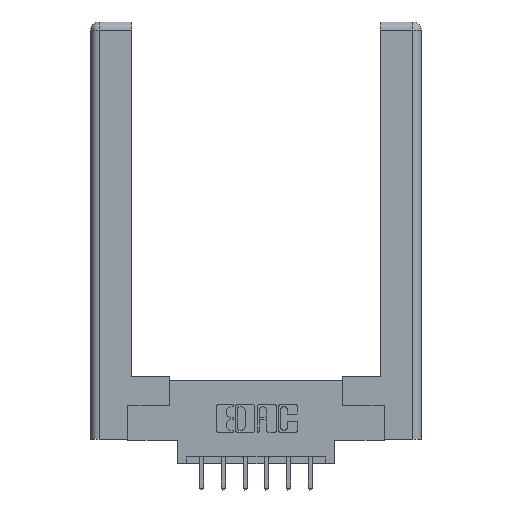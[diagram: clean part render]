
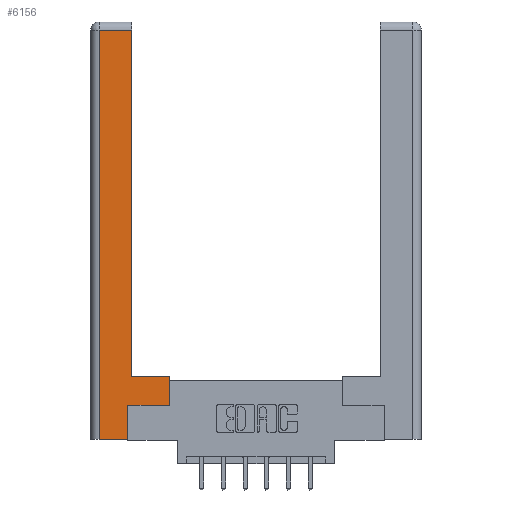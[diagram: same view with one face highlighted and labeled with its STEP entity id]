
A CAD part, top view. The second image highlights one B-rep face of the part: STEP entity #6156.
In plain terms, the highlighted planar face has unit normal (0, 0, 1).
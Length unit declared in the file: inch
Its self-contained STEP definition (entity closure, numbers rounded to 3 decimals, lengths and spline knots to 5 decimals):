
#285 = CARTESIAN_POINT ( 'NONE',  ( 0.565, 0.45, 0. ) ) ;
#335 = VERTEX_POINT ( 'NONE', #6458 ) ;
#541 = EDGE_LOOP ( 'NONE', ( #3999, #8343, #9172, #4169, #6907, #8068, #10866, #2888 ) ) ;
#599 = PLANE ( 'NONE',  #11912 ) ;
#1063 = VERTEX_POINT ( 'NONE', #9950 ) ;
#1333 = LINE ( 'NONE', #1873, #4875 ) ;
#1551 = CARTESIAN_POINT ( 'NONE',  ( 0., 0., 0. ) ) ;
#1620 = LINE ( 'NONE', #5008, #10613 ) ;
#1873 = CARTESIAN_POINT ( 'NONE',  ( 0.265, 0.245, 0. ) ) ;
#1887 = CARTESIAN_POINT ( 'NONE',  ( 0.0615, 0., 0. ) ) ;
#1898 = CARTESIAN_POINT ( 'NONE',  ( 0.565, 0.245, 0. ) ) ;
#2004 = EDGE_CURVE ( 'NONE', #3393, #335, #3284, .T. ) ;
#2440 = VERTEX_POINT ( 'NONE', #8399 ) ;
#2770 = CARTESIAN_POINT ( 'NONE',  ( 0.565, 0.245, 0. ) ) ;
#2888 = ORIENTED_EDGE ( 'NONE', *, *, #11210, .T. ) ;
#2953 = VECTOR ( 'NONE', #6552, 39.37008 ) ;
#2989 = VECTOR ( 'NONE', #7898, 39.37008 ) ;
#3227 = VECTOR ( 'NONE', #10459, 39.37008 ) ;
#3284 = LINE ( 'NONE', #7411, #2989 ) ;
#3364 = VERTEX_POINT ( 'NONE', #2770 ) ;
#3393 = VERTEX_POINT ( 'NONE', #8585 ) ;
#3428 = EDGE_CURVE ( 'NONE', #3364, #9968, #5299, .T. ) ;
#3462 = VECTOR ( 'NONE', #10855, 39.37008 ) ;
#3634 = EDGE_CURVE ( 'NONE', #5063, #2440, #1620, .T. ) ;
#3999 = ORIENTED_EDGE ( 'NONE', *, *, #2004, .T. ) ;
#4094 = DIRECTION ( 'NONE',  ( 1., 0., 0. ) ) ;
#4169 = ORIENTED_EDGE ( 'NONE', *, *, #3634, .T. ) ;
#4875 = VECTOR ( 'NONE', #11137, 39.37008 ) ;
#5008 = CARTESIAN_POINT ( 'NONE',  ( 0.265, 0., 0. ) ) ;
#5063 = VERTEX_POINT ( 'NONE', #1887 ) ;
#5299 = LINE ( 'NONE', #6663, #3227 ) ;
#5358 = CARTESIAN_POINT ( 'NONE',  ( 0.0615, 2.94, 0. ) ) ;
#5493 = FACE_OUTER_BOUND ( 'NONE', #541, .T. ) ;
#5720 = DIRECTION ( 'NONE',  ( 0., -1., 0. ) ) ;
#6040 = LINE ( 'NONE', #1898, #2953 ) ;
#6095 = CARTESIAN_POINT ( 'NONE',  ( 0.295, 0.45, 0. ) ) ;
#6156 = ADVANCED_FACE ( 'NONE', ( #5493 ), #599, .F. ) ;
#6359 = VECTOR ( 'NONE', #6371, 39.37008 ) ;
#6371 = DIRECTION ( 'NONE',  ( -1., 0., 0. ) ) ;
#6458 = CARTESIAN_POINT ( 'NONE',  ( 0.295, 2.94, 0. ) ) ;
#6552 = DIRECTION ( 'NONE',  ( 1., 0., 0. ) ) ;
#6663 = CARTESIAN_POINT ( 'NONE',  ( 0.565, 0.45, 0. ) ) ;
#6907 = ORIENTED_EDGE ( 'NONE', *, *, #11896, .T. ) ;
#7016 = LINE ( 'NONE', #6095, #3462 ) ;
#7411 = CARTESIAN_POINT ( 'NONE',  ( 0.295, 3., 0. ) ) ;
#7898 = DIRECTION ( 'NONE',  ( 0., 1., 0. ) ) ;
#8068 = ORIENTED_EDGE ( 'NONE', *, *, #10869, .T. ) ;
#8343 = ORIENTED_EDGE ( 'NONE', *, *, #10351, .T. ) ;
#8399 = CARTESIAN_POINT ( 'NONE',  ( 0.265, 0., 0. ) ) ;
#8585 = CARTESIAN_POINT ( 'NONE',  ( 0.295, 0.45, 0. ) ) ;
#8929 = DIRECTION ( 'NONE',  ( 0., 0., -1. ) ) ;
#9027 = LINE ( 'NONE', #10482, #11993 ) ;
#9135 = VERTEX_POINT ( 'NONE', #5358 ) ;
#9172 = ORIENTED_EDGE ( 'NONE', *, *, #9348, .T. ) ;
#9348 = EDGE_CURVE ( 'NONE', #9135, #5063, #9027, .T. ) ;
#9950 = CARTESIAN_POINT ( 'NONE',  ( 0.265, 0.245, 0. ) ) ;
#9968 = VERTEX_POINT ( 'NONE', #285 ) ;
#10351 = EDGE_CURVE ( 'NONE', #335, #9135, #11076, .T. ) ;
#10459 = DIRECTION ( 'NONE',  ( 0., 1., 0. ) ) ;
#10482 = CARTESIAN_POINT ( 'NONE',  ( 0.0615, 0., 0. ) ) ;
#10613 = VECTOR ( 'NONE', #4094, 39.37008 ) ;
#10855 = DIRECTION ( 'NONE',  ( -1., 0., 0. ) ) ;
#10866 = ORIENTED_EDGE ( 'NONE', *, *, #3428, .T. ) ;
#10869 = EDGE_CURVE ( 'NONE', #1063, #3364, #6040, .T. ) ;
#11076 = LINE ( 'NONE', #11904, #6359 ) ;
#11137 = DIRECTION ( 'NONE',  ( 0., 1., 0. ) ) ;
#11210 = EDGE_CURVE ( 'NONE', #9968, #3393, #7016, .T. ) ;
#11842 = DIRECTION ( 'NONE',  ( -1., 0., 0. ) ) ;
#11896 = EDGE_CURVE ( 'NONE', #2440, #1063, #1333, .T. ) ;
#11904 = CARTESIAN_POINT ( 'NONE',  ( 0.0615, 2.94, 0. ) ) ;
#11912 = AXIS2_PLACEMENT_3D ( 'NONE', #1551, #8929, #11842 ) ;
#11993 = VECTOR ( 'NONE', #5720, 39.37008 ) ;
